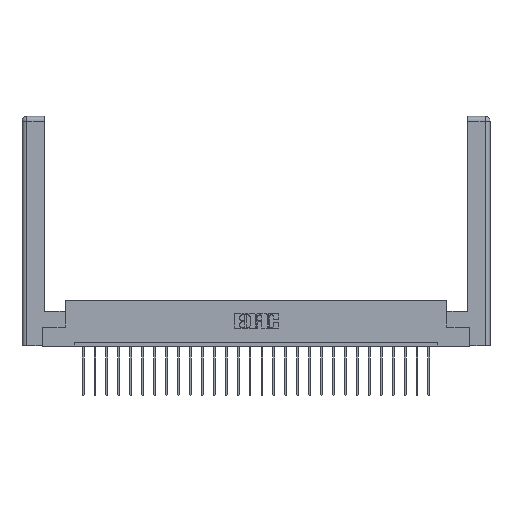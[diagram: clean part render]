
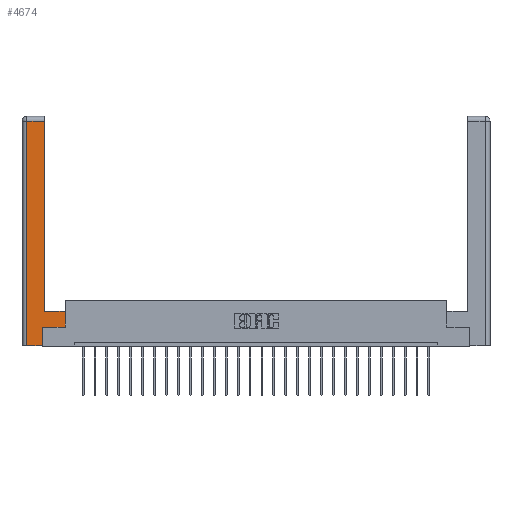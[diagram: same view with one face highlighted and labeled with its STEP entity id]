
A CAD part, top view. The second image highlights one B-rep face of the part: STEP entity #4674.
In plain terms, the highlighted planar face has unit normal (0, 0, 1).
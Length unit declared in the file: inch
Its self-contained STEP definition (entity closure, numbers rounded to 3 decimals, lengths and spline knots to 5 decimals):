
#218 = CARTESIAN_POINT ( 'NONE',  ( 0.0615, 0., 0. ) ) ;
#242 = DIRECTION ( 'NONE',  ( 0., 1., 0. ) ) ;
#368 = CARTESIAN_POINT ( 'NONE',  ( 0., 0., 0. ) ) ;
#1547 = EDGE_CURVE ( 'NONE', #6383, #14357, #19792, .T. ) ;
#2111 = AXIS2_PLACEMENT_3D ( 'NONE', #368, #14392, #4133 ) ;
#2559 = VERTEX_POINT ( 'NONE', #19369 ) ;
#2649 = VERTEX_POINT ( 'NONE', #23588 ) ;
#4133 = DIRECTION ( 'NONE',  ( -1., 0., 0. ) ) ;
#4674 = ADVANCED_FACE ( 'NONE', ( #19931 ), #8244, .F. ) ;
#4739 = DIRECTION ( 'NONE',  ( 0., -1., 0. ) ) ;
#4799 = CARTESIAN_POINT ( 'NONE',  ( 0.295, 0.45, 0. ) ) ;
#6383 = VERTEX_POINT ( 'NONE', #10438 ) ;
#6889 = DIRECTION ( 'NONE',  ( -1., 0., 0. ) ) ;
#6960 = VECTOR ( 'NONE', #21617, 39.37008 ) ;
#7176 = VECTOR ( 'NONE', #22305, 39.37008 ) ;
#7730 = VECTOR ( 'NONE', #18802, 39.37008 ) ;
#7814 = CARTESIAN_POINT ( 'NONE',  ( 0.295, 3., 0. ) ) ;
#8244 = PLANE ( 'NONE',  #2111 ) ;
#8694 = CARTESIAN_POINT ( 'NONE',  ( 0.0615, 0., 0. ) ) ;
#9449 = VECTOR ( 'NONE', #24396, 39.37008 ) ;
#9761 = VECTOR ( 'NONE', #6889, 39.37008 ) ;
#10438 = CARTESIAN_POINT ( 'NONE',  ( 0.565, 0.245, 0. ) ) ;
#10563 = VERTEX_POINT ( 'NONE', #25428 ) ;
#11937 = VECTOR ( 'NONE', #16964, 39.37008 ) ;
#12013 = LINE ( 'NONE', #17031, #9761 ) ;
#12376 = EDGE_CURVE ( 'NONE', #10563, #2559, #25498, .T. ) ;
#13031 = EDGE_CURVE ( 'NONE', #16579, #2649, #19429, .T. ) ;
#13198 = LINE ( 'NONE', #4799, #7730 ) ;
#13960 = ORIENTED_EDGE ( 'NONE', *, *, #19997, .T. ) ;
#14106 = CARTESIAN_POINT ( 'NONE',  ( 0.565, 0.245, 0. ) ) ;
#14357 = VERTEX_POINT ( 'NONE', #16348 ) ;
#14392 = DIRECTION ( 'NONE',  ( 0., 0., -1. ) ) ;
#14556 = LINE ( 'NONE', #23215, #11937 ) ;
#14696 = EDGE_LOOP ( 'NONE', ( #25938, #19877, #13960, #25457, #23094, #22327, #18331, #23904 ) ) ;
#15487 = CARTESIAN_POINT ( 'NONE',  ( 0.265, 0.245, 0. ) ) ;
#16011 = CARTESIAN_POINT ( 'NONE',  ( 0.295, 0.45, 0. ) ) ;
#16348 = CARTESIAN_POINT ( 'NONE',  ( 0.565, 0.45, 0. ) ) ;
#16579 = VERTEX_POINT ( 'NONE', #16011 ) ;
#16914 = LINE ( 'NONE', #8694, #22023 ) ;
#16964 = DIRECTION ( 'NONE',  ( 1., 0., 0. ) ) ;
#17031 = CARTESIAN_POINT ( 'NONE',  ( 0.0615, 2.94, 0. ) ) ;
#18331 = ORIENTED_EDGE ( 'NONE', *, *, #1547, .T. ) ;
#18802 = DIRECTION ( 'NONE',  ( -1., 0., 0. ) ) ;
#18877 = VERTEX_POINT ( 'NONE', #24489 ) ;
#19025 = VERTEX_POINT ( 'NONE', #218 ) ;
#19369 = CARTESIAN_POINT ( 'NONE',  ( 0.265, 0.245, 0. ) ) ;
#19429 = LINE ( 'NONE', #7814, #9449 ) ;
#19792 = LINE ( 'NONE', #21923, #23934 ) ;
#19877 = ORIENTED_EDGE ( 'NONE', *, *, #21531, .T. ) ;
#19931 = FACE_OUTER_BOUND ( 'NONE', #14696, .T. ) ;
#19997 = EDGE_CURVE ( 'NONE', #18877, #19025, #16914, .T. ) ;
#21531 = EDGE_CURVE ( 'NONE', #2649, #18877, #12013, .T. ) ;
#21617 = DIRECTION ( 'NONE',  ( 0., 1., 0. ) ) ;
#21923 = CARTESIAN_POINT ( 'NONE',  ( 0.565, 0.45, 0. ) ) ;
#22023 = VECTOR ( 'NONE', #4739, 39.37008 ) ;
#22305 = DIRECTION ( 'NONE',  ( 1., 0., 0. ) ) ;
#22327 = ORIENTED_EDGE ( 'NONE', *, *, #26284, .T. ) ;
#23071 = EDGE_CURVE ( 'NONE', #14357, #16579, #13198, .T. ) ;
#23094 = ORIENTED_EDGE ( 'NONE', *, *, #12376, .T. ) ;
#23215 = CARTESIAN_POINT ( 'NONE',  ( 0.265, 0., 0. ) ) ;
#23531 = LINE ( 'NONE', #14106, #7176 ) ;
#23588 = CARTESIAN_POINT ( 'NONE',  ( 0.295, 2.94, 0. ) ) ;
#23904 = ORIENTED_EDGE ( 'NONE', *, *, #23071, .T. ) ;
#23934 = VECTOR ( 'NONE', #242, 39.37008 ) ;
#24135 = EDGE_CURVE ( 'NONE', #19025, #10563, #14556, .T. ) ;
#24396 = DIRECTION ( 'NONE',  ( 0., 1., 0. ) ) ;
#24489 = CARTESIAN_POINT ( 'NONE',  ( 0.0615, 2.94, 0. ) ) ;
#25428 = CARTESIAN_POINT ( 'NONE',  ( 0.265, 0., 0. ) ) ;
#25457 = ORIENTED_EDGE ( 'NONE', *, *, #24135, .T. ) ;
#25498 = LINE ( 'NONE', #15487, #6960 ) ;
#25938 = ORIENTED_EDGE ( 'NONE', *, *, #13031, .T. ) ;
#26284 = EDGE_CURVE ( 'NONE', #2559, #6383, #23531, .T. ) ;
